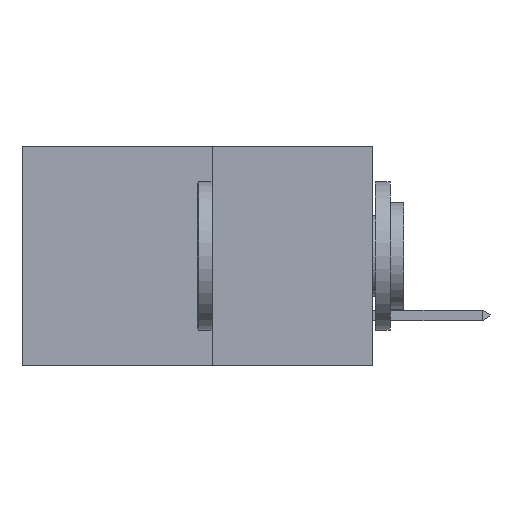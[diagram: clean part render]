
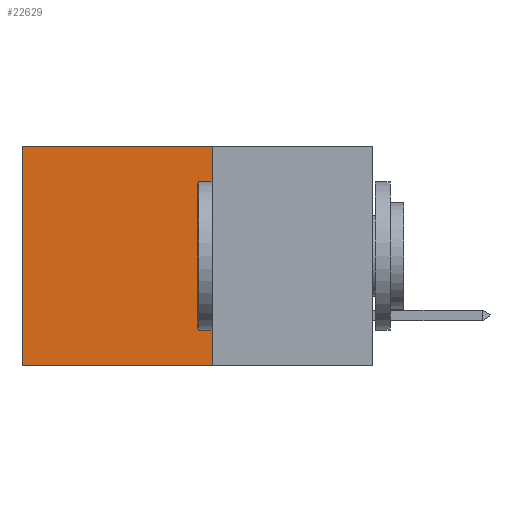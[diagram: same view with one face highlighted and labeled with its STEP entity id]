
A CAD part, left-side view. The second image highlights one B-rep face of the part: STEP entity #22629.
In plain terms, the highlighted planar face has unit normal (-1, 0, 0).
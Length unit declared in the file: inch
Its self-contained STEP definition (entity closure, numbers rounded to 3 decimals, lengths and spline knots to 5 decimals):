
#29 = EDGE_CURVE ( 'NONE', #27189, #25006, #25957, .T. ) ;
#4008 = ORIENTED_EDGE ( 'NONE', *, *, #29, .F. ) ;
#5189 = EDGE_CURVE ( 'NONE', #25006, #24114, #19552, .T. ) ;
#5290 = CARTESIAN_POINT ( 'NONE',  ( 0.277, 0.27, -0.37 ) ) ;
#6597 = VECTOR ( 'NONE', #16123, 39.37008 ) ;
#7770 = EDGE_CURVE ( 'NONE', #22715, #24114, #17367, .T. ) ;
#8039 = CARTESIAN_POINT ( 'NONE',  ( 0.277, 0.59, 0. ) ) ;
#8217 = DIRECTION ( 'NONE',  ( 0., 1., 0. ) ) ;
#8261 = CARTESIAN_POINT ( 'NONE',  ( 0.277, 0.59, -0.37 ) ) ;
#10492 = AXIS2_PLACEMENT_3D ( 'NONE', #5290, #12893, #30475 ) ;
#11602 = ORIENTED_EDGE ( 'NONE', *, *, #7770, .T. ) ;
#12276 = VECTOR ( 'NONE', #18232, 39.37008 ) ;
#12443 = VECTOR ( 'NONE', #8217, 39.37008 ) ;
#12893 = DIRECTION ( 'NONE',  ( 1., 0., 0. ) ) ;
#12903 = VECTOR ( 'NONE', #13117, 39.37008 ) ;
#13117 = DIRECTION ( 'NONE',  ( 0., 1., 0. ) ) ;
#13219 = CARTESIAN_POINT ( 'NONE',  ( 0.277, 0.27, -0.37 ) ) ;
#15862 = CARTESIAN_POINT ( 'NONE',  ( 0.277, 0.27, -0.37 ) ) ;
#16123 = DIRECTION ( 'NONE',  ( 0., 0., -1. ) ) ;
#17367 = LINE ( 'NONE', #8261, #12276 ) ;
#18232 = DIRECTION ( 'NONE',  ( 0., 0., -1. ) ) ;
#19083 = LINE ( 'NONE', #25859, #12443 ) ;
#19552 = LINE ( 'NONE', #13219, #12903 ) ;
#20231 = CARTESIAN_POINT ( 'NONE',  ( 0.277, 0.27, 0. ) ) ;
#21957 = ORIENTED_EDGE ( 'NONE', *, *, #26135, .T. ) ;
#22099 = EDGE_LOOP ( 'NONE', ( #11602, #31912, #4008, #21957 ) ) ;
#22629 = ADVANCED_FACE ( 'NONE', ( #24027 ), #27982, .F. ) ;
#22715 = VERTEX_POINT ( 'NONE', #8039 ) ;
#24027 = FACE_OUTER_BOUND ( 'NONE', #22099, .T. ) ;
#24114 = VERTEX_POINT ( 'NONE', #25928 ) ;
#25006 = VERTEX_POINT ( 'NONE', #27426 ) ;
#25859 = CARTESIAN_POINT ( 'NONE',  ( 0.277, 0.27, 0. ) ) ;
#25928 = CARTESIAN_POINT ( 'NONE',  ( 0.277, 0.59, -0.37 ) ) ;
#25957 = LINE ( 'NONE', #15862, #6597 ) ;
#26135 = EDGE_CURVE ( 'NONE', #27189, #22715, #19083, .T. ) ;
#27189 = VERTEX_POINT ( 'NONE', #20231 ) ;
#27426 = CARTESIAN_POINT ( 'NONE',  ( 0.277, 0.27, -0.37 ) ) ;
#27982 = PLANE ( 'NONE',  #10492 ) ;
#30475 = DIRECTION ( 'NONE',  ( 0., 0., -1. ) ) ;
#31912 = ORIENTED_EDGE ( 'NONE', *, *, #5189, .F. ) ;
